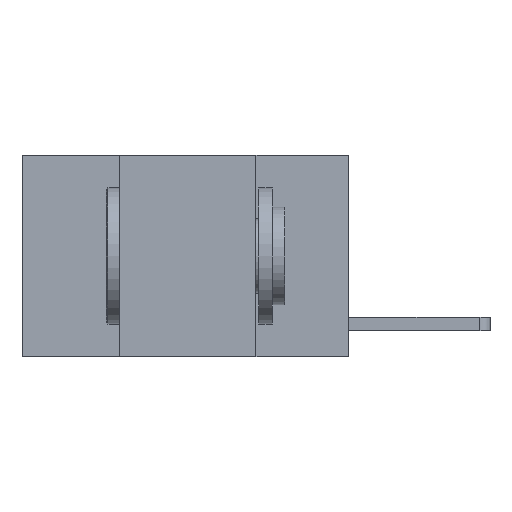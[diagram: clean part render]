
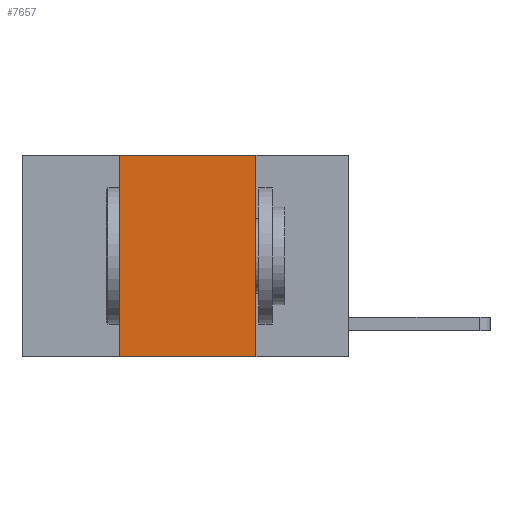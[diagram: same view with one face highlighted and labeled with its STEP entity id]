
A CAD part, left-side view. The second image highlights one B-rep face of the part: STEP entity #7657.
In plain terms, the highlighted planar face has unit normal (-1, 0, 0).
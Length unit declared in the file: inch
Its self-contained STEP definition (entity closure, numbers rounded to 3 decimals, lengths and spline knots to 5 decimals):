
#190 = LINE ( 'NONE', #3607, #10241 ) ;
#861 = DIRECTION ( 'NONE',  ( 0., -1., 0. ) ) ;
#1020 = DIRECTION ( 'NONE',  ( 0., 0., -1. ) ) ;
#1246 = VERTEX_POINT ( 'NONE', #2886 ) ;
#1342 = CARTESIAN_POINT ( 'NONE',  ( 0., 0.6, -0.37 ) ) ;
#1494 = EDGE_CURVE ( 'NONE', #1246, #6717, #2093, .T. ) ;
#1861 = VECTOR ( 'NONE', #9132, 39.37008 ) ;
#1881 = EDGE_LOOP ( 'NONE', ( #2281, #2295, #2420, #2519 ) ) ;
#2093 = LINE ( 'NONE', #1342, #1861 ) ;
#2281 = ORIENTED_EDGE ( 'NONE', *, *, #9752, .F. ) ;
#2295 = ORIENTED_EDGE ( 'NONE', *, *, #6883, .F. ) ;
#2420 = ORIENTED_EDGE ( 'NONE', *, *, #8916, .F. ) ;
#2519 = ORIENTED_EDGE ( 'NONE', *, *, #1494, .T. ) ;
#2715 = CARTESIAN_POINT ( 'NONE',  ( 0., 0.17, 0. ) ) ;
#2886 = CARTESIAN_POINT ( 'NONE',  ( 0., 0.42, -0.37 ) ) ;
#3607 = CARTESIAN_POINT ( 'NONE',  ( 0., 0.17, 0. ) ) ;
#3926 = CARTESIAN_POINT ( 'NONE',  ( 0., 0.42, 0. ) ) ;
#4413 = DIRECTION ( 'NONE',  ( 0., 0., -1. ) ) ;
#5006 = CARTESIAN_POINT ( 'NONE',  ( 0., 0.6, 0. ) ) ;
#5189 = FACE_OUTER_BOUND ( 'NONE', #1881, .T. ) ;
#5664 = VECTOR ( 'NONE', #8914, 39.37008 ) ;
#5708 = CARTESIAN_POINT ( 'NONE',  ( 0., 0.42, 0. ) ) ;
#5797 = DIRECTION ( 'NONE',  ( 1., 0., 0. ) ) ;
#6207 = CARTESIAN_POINT ( 'NONE',  ( 0., 0.17, -0.37 ) ) ;
#6717 = VERTEX_POINT ( 'NONE', #6207 ) ;
#6883 = EDGE_CURVE ( 'NONE', #9330, #9724, #9815, .T. ) ;
#7657 = ADVANCED_FACE ( 'NONE', ( #5189 ), #9771, .F. ) ;
#8914 = DIRECTION ( 'NONE',  ( 0., 0., 1. ) ) ;
#8916 = EDGE_CURVE ( 'NONE', #1246, #9330, #9899, .T. ) ;
#9132 = DIRECTION ( 'NONE',  ( 0., -1., 0. ) ) ;
#9297 = AXIS2_PLACEMENT_3D ( 'NONE', #5006, #5797, #1020 ) ;
#9330 = VERTEX_POINT ( 'NONE', #3926 ) ;
#9585 = VECTOR ( 'NONE', #861, 39.37008 ) ;
#9645 = CARTESIAN_POINT ( 'NONE',  ( 0., 0.6, 0. ) ) ;
#9724 = VERTEX_POINT ( 'NONE', #2715 ) ;
#9752 = EDGE_CURVE ( 'NONE', #9724, #6717, #190, .T. ) ;
#9771 = PLANE ( 'NONE',  #9297 ) ;
#9815 = LINE ( 'NONE', #9645, #9585 ) ;
#9899 = LINE ( 'NONE', #5708, #5664 ) ;
#10241 = VECTOR ( 'NONE', #4413, 39.37008 ) ;
